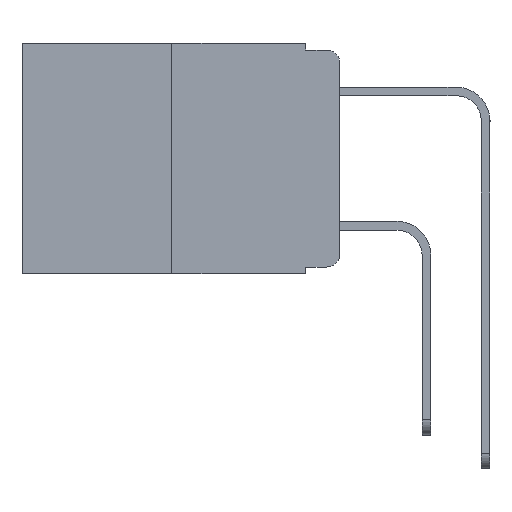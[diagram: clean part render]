
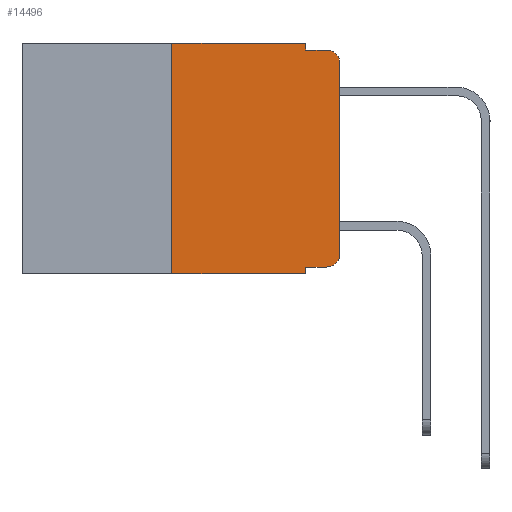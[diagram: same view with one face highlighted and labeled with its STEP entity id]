
A CAD part, left-side view. The second image highlights one B-rep face of the part: STEP entity #14496.
In plain terms, the highlighted planar face has unit normal (-1, 0, 0).
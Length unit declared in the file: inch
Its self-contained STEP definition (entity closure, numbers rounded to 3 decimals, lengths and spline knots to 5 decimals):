
#187 = DIRECTION ( 'NONE',  ( 0., 0., -1. ) ) ;
#295 = CARTESIAN_POINT ( 'NONE',  ( 0., 0.051, -0.01 ) ) ;
#329 = EDGE_CURVE ( 'NONE', #16198, #6082, #2584, .T. ) ;
#375 = CARTESIAN_POINT ( 'NONE',  ( 0., 0.473, 0. ) ) ;
#498 = VECTOR ( 'NONE', #4110, 39.37008 ) ;
#897 = VERTEX_POINT ( 'NONE', #19146 ) ;
#1099 = LINE ( 'NONE', #14839, #498 ) ;
#1543 = EDGE_CURVE ( 'NONE', #21710, #16989, #10220, .T. ) ;
#1575 = AXIS2_PLACEMENT_3D ( 'NONE', #2416, #15030, #4308 ) ;
#1699 = ORIENTED_EDGE ( 'NONE', *, *, #6974, .T. ) ;
#1727 = EDGE_CURVE ( 'NONE', #16989, #22181, #21458, .T. ) ;
#2416 = CARTESIAN_POINT ( 'NONE',  ( 0., 0.02, -0.313 ) ) ;
#2584 = LINE ( 'NONE', #375, #16343 ) ;
#4044 = LINE ( 'NONE', #11220, #22271 ) ;
#4110 = DIRECTION ( 'NONE',  ( 0., -1., 0. ) ) ;
#4308 = DIRECTION ( 'NONE',  ( 0., 0., -1. ) ) ;
#4541 = VERTEX_POINT ( 'NONE', #7474 ) ;
#4658 = VECTOR ( 'NONE', #21507, 39.37008 ) ;
#5133 = CARTESIAN_POINT ( 'NONE',  ( 0., 0.02, -0.03 ) ) ;
#5430 = VECTOR ( 'NONE', #15140, 39.37008 ) ;
#5444 = ORIENTED_EDGE ( 'NONE', *, *, #12046, .F. ) ;
#5521 = VECTOR ( 'NONE', #7746, 39.37008 ) ;
#6013 = ORIENTED_EDGE ( 'NONE', *, *, #1727, .T. ) ;
#6082 = VERTEX_POINT ( 'NONE', #10285 ) ;
#6588 = VERTEX_POINT ( 'NONE', #8166 ) ;
#6974 = EDGE_CURVE ( 'NONE', #4541, #10149, #9424, .T. ) ;
#7062 = VERTEX_POINT ( 'NONE', #295 ) ;
#7223 = CARTESIAN_POINT ( 'NONE',  ( 0., 0., -0.313 ) ) ;
#7474 = CARTESIAN_POINT ( 'NONE',  ( 0., 0.051, -0.333 ) ) ;
#7702 = LINE ( 'NONE', #23099, #21251 ) ;
#7736 = CARTESIAN_POINT ( 'NONE',  ( 0., 0.25, 0. ) ) ;
#7746 = DIRECTION ( 'NONE',  ( 0., 0., -1. ) ) ;
#8166 = CARTESIAN_POINT ( 'NONE',  ( 0., 0.051, -0.343 ) ) ;
#8251 = ORIENTED_EDGE ( 'NONE', *, *, #329, .F. ) ;
#8322 = LINE ( 'NONE', #9076, #20763 ) ;
#8501 = CARTESIAN_POINT ( 'NONE',  ( 0., 0., -0.03 ) ) ;
#9076 = CARTESIAN_POINT ( 'NONE',  ( 0., 0.25, 0. ) ) ;
#9109 = ORIENTED_EDGE ( 'NONE', *, *, #1543, .T. ) ;
#9393 = EDGE_CURVE ( 'NONE', #897, #16198, #8322, .T. ) ;
#9424 = LINE ( 'NONE', #11073, #4658 ) ;
#9580 = EDGE_CURVE ( 'NONE', #10149, #21710, #12343, .T. ) ;
#9976 = DIRECTION ( 'NONE',  ( 0., 0., -1. ) ) ;
#10149 = VERTEX_POINT ( 'NONE', #20248 ) ;
#10220 = LINE ( 'NONE', #19950, #5430 ) ;
#10285 = CARTESIAN_POINT ( 'NONE',  ( 0., 0.051, 0. ) ) ;
#10798 = CARTESIAN_POINT ( 'NONE',  ( 0., 0.02, -0.01 ) ) ;
#10862 = ORIENTED_EDGE ( 'NONE', *, *, #22896, .F. ) ;
#10969 = AXIS2_PLACEMENT_3D ( 'NONE', #5133, #19724, #19252 ) ;
#11073 = CARTESIAN_POINT ( 'NONE',  ( 0., 0.051, -0.333 ) ) ;
#11220 = CARTESIAN_POINT ( 'NONE',  ( 0., 0.051, 0. ) ) ;
#12046 = EDGE_CURVE ( 'NONE', #4541, #6588, #4044, .T. ) ;
#12343 = CIRCLE ( 'NONE', #1575, 0.02 ) ;
#13578 = FACE_OUTER_BOUND ( 'NONE', #17435, .T. ) ;
#13785 = DIRECTION ( 'NONE',  ( 0., -1., 0. ) ) ;
#14496 = ADVANCED_FACE ( 'NONE', ( #13578 ), #15279, .F. ) ;
#14839 = CARTESIAN_POINT ( 'NONE',  ( 0., 0.473, -0.343 ) ) ;
#15030 = DIRECTION ( 'NONE',  ( -1., 0., 0. ) ) ;
#15053 = LINE ( 'NONE', #16645, #5521 ) ;
#15140 = DIRECTION ( 'NONE',  ( 0., 0., 1. ) ) ;
#15279 = PLANE ( 'NONE',  #20777 ) ;
#16198 = VERTEX_POINT ( 'NONE', #7736 ) ;
#16297 = DIRECTION ( 'NONE',  ( 0., -1., 0. ) ) ;
#16343 = VECTOR ( 'NONE', #13785, 39.37008 ) ;
#16645 = CARTESIAN_POINT ( 'NONE',  ( 0., 0.051, 0. ) ) ;
#16989 = VERTEX_POINT ( 'NONE', #8501 ) ;
#17029 = CARTESIAN_POINT ( 'NONE',  ( 0., 0.473, 0. ) ) ;
#17435 = EDGE_LOOP ( 'NONE', ( #9109, #6013, #10862, #20700, #8251, #17978, #18525, #5444, #1699, #21216 ) ) ;
#17978 = ORIENTED_EDGE ( 'NONE', *, *, #9393, .F. ) ;
#17994 = EDGE_CURVE ( 'NONE', #6082, #7062, #15053, .T. ) ;
#18525 = ORIENTED_EDGE ( 'NONE', *, *, #19928, .T. ) ;
#19146 = CARTESIAN_POINT ( 'NONE',  ( 0., 0.25, -0.343 ) ) ;
#19252 = DIRECTION ( 'NONE',  ( 0., 0., -1. ) ) ;
#19671 = DIRECTION ( 'NONE',  ( 0., 0., 1. ) ) ;
#19724 = DIRECTION ( 'NONE',  ( -1., 0., 0. ) ) ;
#19928 = EDGE_CURVE ( 'NONE', #897, #6588, #1099, .T. ) ;
#19950 = CARTESIAN_POINT ( 'NONE',  ( 0., 0., 0. ) ) ;
#20248 = CARTESIAN_POINT ( 'NONE',  ( 0., 0.02, -0.333 ) ) ;
#20516 = DIRECTION ( 'NONE',  ( 1., 0., 0. ) ) ;
#20700 = ORIENTED_EDGE ( 'NONE', *, *, #17994, .F. ) ;
#20763 = VECTOR ( 'NONE', #19671, 39.37008 ) ;
#20777 = AXIS2_PLACEMENT_3D ( 'NONE', #17029, #20516, #9976 ) ;
#21216 = ORIENTED_EDGE ( 'NONE', *, *, #9580, .T. ) ;
#21251 = VECTOR ( 'NONE', #16297, 39.37008 ) ;
#21458 = CIRCLE ( 'NONE', #10969, 0.02 ) ;
#21507 = DIRECTION ( 'NONE',  ( 0., -1., 0. ) ) ;
#21710 = VERTEX_POINT ( 'NONE', #7223 ) ;
#22181 = VERTEX_POINT ( 'NONE', #10798 ) ;
#22271 = VECTOR ( 'NONE', #187, 39.37008 ) ;
#22896 = EDGE_CURVE ( 'NONE', #7062, #22181, #7702, .T. ) ;
#23099 = CARTESIAN_POINT ( 'NONE',  ( 0., 0.051, -0.01 ) ) ;
